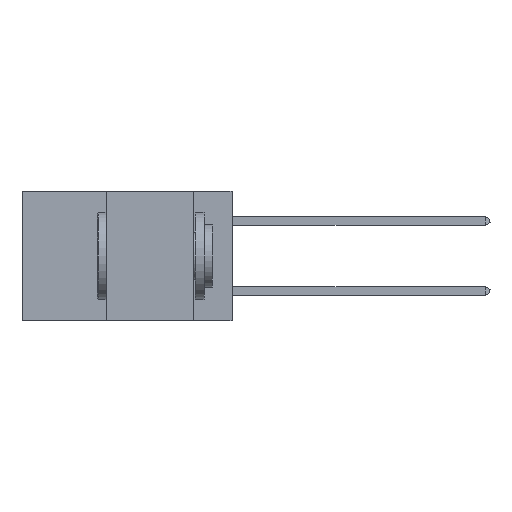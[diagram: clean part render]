
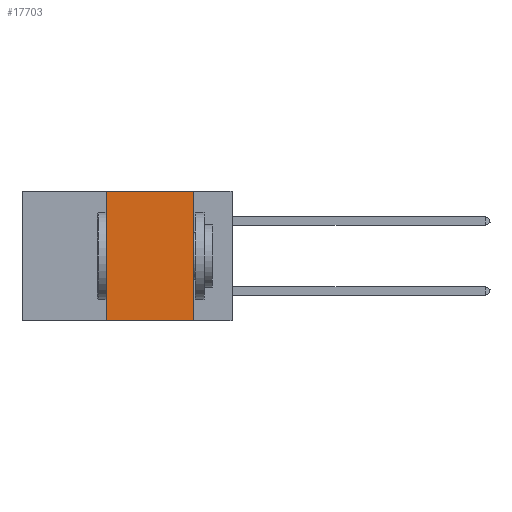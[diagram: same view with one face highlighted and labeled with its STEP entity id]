
A CAD part, left-side view. The second image highlights one B-rep face of the part: STEP entity #17703.
In plain terms, the highlighted planar face has unit normal (-1, 0, 0).
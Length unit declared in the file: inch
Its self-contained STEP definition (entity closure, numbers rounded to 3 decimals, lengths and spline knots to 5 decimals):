
#1081 = DIRECTION ( 'NONE',  ( 0., -1., 0. ) ) ;
#1341 = DIRECTION ( 'NONE',  ( 0., -1., 0. ) ) ;
#3194 = EDGE_CURVE ( 'NONE', #22100, #9354, #28241, .T. ) ;
#3547 = PLANE ( 'NONE',  #9081 ) ;
#3653 = VERTEX_POINT ( 'NONE', #28467 ) ;
#6188 = DIRECTION ( 'NONE',  ( 0., 0., -1. ) ) ;
#6337 = VECTOR ( 'NONE', #1341, 39.37008 ) ;
#7296 = VECTOR ( 'NONE', #24184, 39.37008 ) ;
#7845 = DIRECTION ( 'NONE',  ( 0., 0., -1. ) ) ;
#8343 = CARTESIAN_POINT ( 'NONE',  ( 0., 0.36, 0. ) ) ;
#9081 = AXIS2_PLACEMENT_3D ( 'NONE', #16371, #21352, #6188 ) ;
#9354 = VERTEX_POINT ( 'NONE', #8343 ) ;
#10042 = ORIENTED_EDGE ( 'NONE', *, *, #19851, .F. ) ;
#10767 = EDGE_CURVE ( 'NONE', #22100, #29837, #24961, .T. ) ;
#12144 = VECTOR ( 'NONE', #7845, 39.37008 ) ;
#14217 = CARTESIAN_POINT ( 'NONE',  ( 0., 0.6, 0. ) ) ;
#14724 = CARTESIAN_POINT ( 'NONE',  ( 0., 0.36, -0.37 ) ) ;
#16371 = CARTESIAN_POINT ( 'NONE',  ( 0., 0.6, 0. ) ) ;
#16679 = CARTESIAN_POINT ( 'NONE',  ( 0., 0.36, 0. ) ) ;
#17703 = ADVANCED_FACE ( 'NONE', ( #19359 ), #3547, .F. ) ;
#18138 = EDGE_LOOP ( 'NONE', ( #29316, #10042, #21875, #29737 ) ) ;
#19046 = CARTESIAN_POINT ( 'NONE',  ( 0., 0.6, -0.37 ) ) ;
#19122 = VECTOR ( 'NONE', #1081, 39.37008 ) ;
#19359 = FACE_OUTER_BOUND ( 'NONE', #18138, .T. ) ;
#19851 = EDGE_CURVE ( 'NONE', #9354, #3653, #25686, .T. ) ;
#21352 = DIRECTION ( 'NONE',  ( 1., 0., 0. ) ) ;
#21409 = CARTESIAN_POINT ( 'NONE',  ( 0., 0.11, -0.37 ) ) ;
#21875 = ORIENTED_EDGE ( 'NONE', *, *, #3194, .F. ) ;
#22100 = VERTEX_POINT ( 'NONE', #14724 ) ;
#22965 = CARTESIAN_POINT ( 'NONE',  ( 0., 0.11, 0. ) ) ;
#22999 = EDGE_CURVE ( 'NONE', #3653, #29837, #24728, .T. ) ;
#24184 = DIRECTION ( 'NONE',  ( 0., 0., 1. ) ) ;
#24728 = LINE ( 'NONE', #22965, #12144 ) ;
#24961 = LINE ( 'NONE', #19046, #19122 ) ;
#25686 = LINE ( 'NONE', #14217, #6337 ) ;
#28241 = LINE ( 'NONE', #16679, #7296 ) ;
#28467 = CARTESIAN_POINT ( 'NONE',  ( 0., 0.11, 0. ) ) ;
#29316 = ORIENTED_EDGE ( 'NONE', *, *, #22999, .F. ) ;
#29737 = ORIENTED_EDGE ( 'NONE', *, *, #10767, .T. ) ;
#29837 = VERTEX_POINT ( 'NONE', #21409 ) ;
